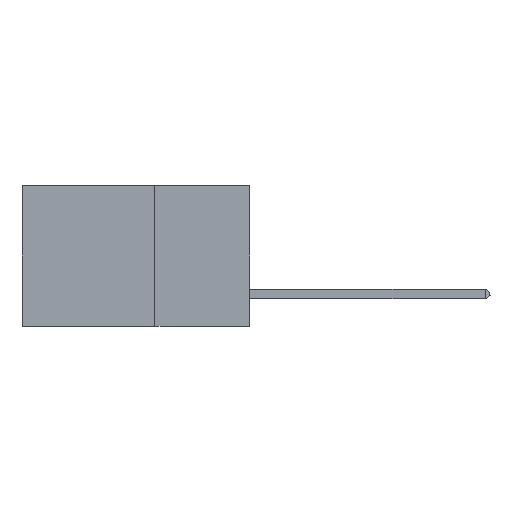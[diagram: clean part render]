
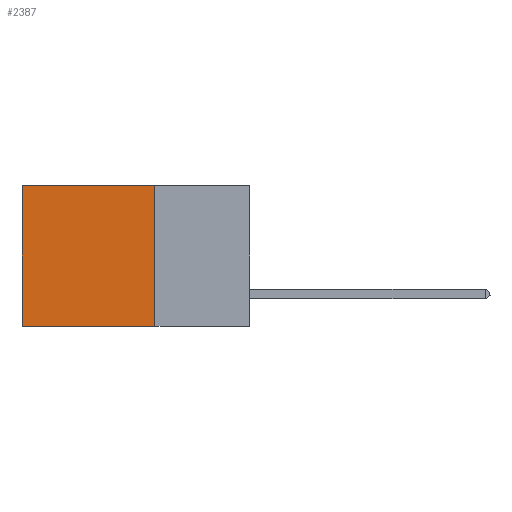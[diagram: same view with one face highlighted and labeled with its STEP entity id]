
A CAD part, left-side view. The second image highlights one B-rep face of the part: STEP entity #2387.
In plain terms, the highlighted planar face has unit normal (-1, 0, 0).
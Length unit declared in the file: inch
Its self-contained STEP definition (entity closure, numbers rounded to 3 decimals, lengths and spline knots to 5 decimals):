
#78 = AXIS2_PLACEMENT_3D ( 'NONE', #24305, #29114, #775 ) ;
#524 = LINE ( 'NONE', #22068, #3918 ) ;
#775 = DIRECTION ( 'NONE',  ( 0., 0., -1. ) ) ;
#893 = LINE ( 'NONE', #27366, #28585 ) ;
#1701 = EDGE_LOOP ( 'NONE', ( #20510, #13105, #21368, #7601 ) ) ;
#2387 = ADVANCED_FACE ( 'NONE', ( #12661 ), #19528, .F. ) ;
#3918 = VECTOR ( 'NONE', #22261, 39.37008 ) ;
#7601 = ORIENTED_EDGE ( 'NONE', *, *, #22684, .T. ) ;
#8152 = CARTESIAN_POINT ( 'NONE',  ( 0.2875, 0.6, -0.37 ) ) ;
#9185 = VERTEX_POINT ( 'NONE', #14554 ) ;
#12619 = VECTOR ( 'NONE', #29140, 39.37008 ) ;
#12661 = FACE_OUTER_BOUND ( 'NONE', #1701, .T. ) ;
#13071 = DIRECTION ( 'NONE',  ( 0., 1., 0. ) ) ;
#13105 = ORIENTED_EDGE ( 'NONE', *, *, #22455, .F. ) ;
#14554 = CARTESIAN_POINT ( 'NONE',  ( 0.2875, 0.6, 0. ) ) ;
#15512 = VERTEX_POINT ( 'NONE', #22037 ) ;
#19528 = PLANE ( 'NONE',  #78 ) ;
#20510 = ORIENTED_EDGE ( 'NONE', *, *, #27620, .T. ) ;
#21368 = ORIENTED_EDGE ( 'NONE', *, *, #21543, .F. ) ;
#21543 = EDGE_CURVE ( 'NONE', #24195, #15512, #22306, .T. ) ;
#22037 = CARTESIAN_POINT ( 'NONE',  ( 0.2875, 0.25, -0.37 ) ) ;
#22068 = CARTESIAN_POINT ( 'NONE',  ( 0.2875, 0.25, -0.37 ) ) ;
#22261 = DIRECTION ( 'NONE',  ( 0., 1., 0. ) ) ;
#22306 = LINE ( 'NONE', #26757, #12619 ) ;
#22387 = VERTEX_POINT ( 'NONE', #8152 ) ;
#22455 = EDGE_CURVE ( 'NONE', #15512, #22387, #524, .T. ) ;
#22684 = EDGE_CURVE ( 'NONE', #24195, #9185, #893, .T. ) ;
#22940 = LINE ( 'NONE', #27631, #24076 ) ;
#24076 = VECTOR ( 'NONE', #30038, 39.37008 ) ;
#24195 = VERTEX_POINT ( 'NONE', #29771 ) ;
#24305 = CARTESIAN_POINT ( 'NONE',  ( 0.2875, 0.25, 0. ) ) ;
#26757 = CARTESIAN_POINT ( 'NONE',  ( 0.2875, 0.25, 0. ) ) ;
#27366 = CARTESIAN_POINT ( 'NONE',  ( 0.2875, 0.25, 0. ) ) ;
#27620 = EDGE_CURVE ( 'NONE', #9185, #22387, #22940, .T. ) ;
#27631 = CARTESIAN_POINT ( 'NONE',  ( 0.2875, 0.6, 0. ) ) ;
#28585 = VECTOR ( 'NONE', #13071, 39.37008 ) ;
#29114 = DIRECTION ( 'NONE',  ( 1., 0., 0. ) ) ;
#29140 = DIRECTION ( 'NONE',  ( 0., 0., -1. ) ) ;
#29771 = CARTESIAN_POINT ( 'NONE',  ( 0.2875, 0.25, 0. ) ) ;
#30038 = DIRECTION ( 'NONE',  ( 0., 0., -1. ) ) ;
